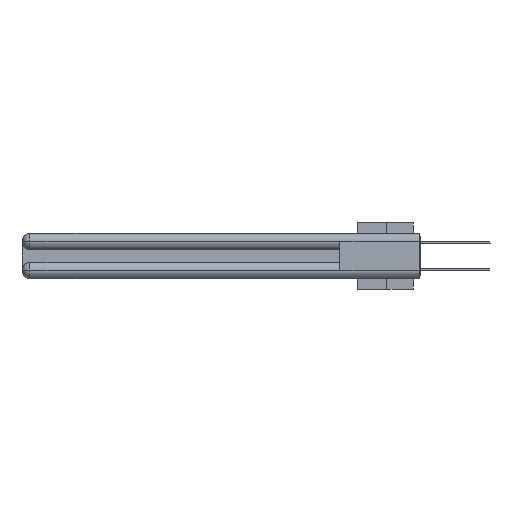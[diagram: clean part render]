
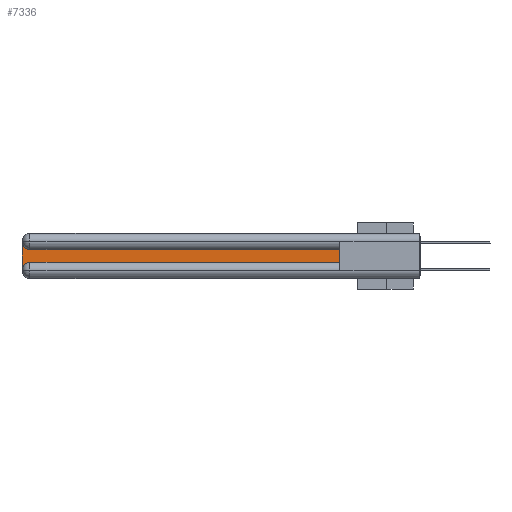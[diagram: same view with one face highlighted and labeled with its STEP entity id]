
A CAD part, left-side view. The second image highlights one B-rep face of the part: STEP entity #7336.
In plain terms, the highlighted planar face has unit normal (-1, 0, 0).
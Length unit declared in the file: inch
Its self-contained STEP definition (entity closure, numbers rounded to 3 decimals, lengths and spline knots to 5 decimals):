
#3 = DIRECTION ( 'NONE',  ( 0., 0., 1. ) ) ;
#573 = DIRECTION ( 'NONE',  ( 0., 1., 0. ) ) ;
#1075 = LINE ( 'NONE', #16398, #37782 ) ;
#2885 = DIRECTION ( 'NONE',  ( 0., 0., -1. ) ) ;
#3100 = DIRECTION ( 'NONE',  ( 1., 0., 0. ) ) ;
#4348 = LINE ( 'NONE', #16305, #14561 ) ;
#4958 = EDGE_CURVE ( 'NONE', #39099, #21110, #28471, .T. ) ;
#5521 = DIRECTION ( 'NONE',  ( 0., 0., -1. ) ) ;
#5944 = DIRECTION ( 'NONE',  ( 1., 0., 0. ) ) ;
#6225 = CARTESIAN_POINT ( 'NONE',  ( 0.075, 2.94, -0.2775 ) ) ;
#7336 = ADVANCED_FACE ( 'NONE', ( #25384 ), #31634, .F. ) ;
#8927 = VECTOR ( 'NONE', #3, 39.37008 ) ;
#10558 = CARTESIAN_POINT ( 'NONE',  ( 0.075, 0.6, -0.2175 ) ) ;
#14336 = EDGE_CURVE ( 'NONE', #37488, #26446, #1075, .T. ) ;
#14561 = VECTOR ( 'NONE', #573, 39.37008 ) ;
#15164 = VECTOR ( 'NONE', #25741, 39.37008 ) ;
#16305 = CARTESIAN_POINT ( 'NONE',  ( 0.075, 0.6, -0.1225 ) ) ;
#16398 = CARTESIAN_POINT ( 'NONE',  ( 0.075, 0.6, -0.2175 ) ) ;
#16841 = EDGE_CURVE ( 'NONE', #24533, #39099, #22353, .T. ) ;
#17554 = AXIS2_PLACEMENT_3D ( 'NONE', #6225, #3100, #20787 ) ;
#17930 = CARTESIAN_POINT ( 'NONE',  ( 0.075, 2.94, -0.0625 ) ) ;
#18009 = EDGE_CURVE ( 'NONE', #19105, #24533, #4348, .T. ) ;
#18249 = ORIENTED_EDGE ( 'NONE', *, *, #37626, .T. ) ;
#18972 = AXIS2_PLACEMENT_3D ( 'NONE', #17930, #5944, #5521 ) ;
#19105 = VERTEX_POINT ( 'NONE', #32090 ) ;
#19639 = CARTESIAN_POINT ( 'NONE',  ( 0.075, 3., -0.2775 ) ) ;
#19967 = CARTESIAN_POINT ( 'NONE',  ( 0.075, 2.94, -0.2175 ) ) ;
#20294 = AXIS2_PLACEMENT_3D ( 'NONE', #24542, #21560, #2885 ) ;
#20787 = DIRECTION ( 'NONE',  ( 0., 0., -1. ) ) ;
#20843 = EDGE_LOOP ( 'NONE', ( #36599, #25757, #38647, #18249, #28880, #35596 ) ) ;
#21110 = VERTEX_POINT ( 'NONE', #19639 ) ;
#21560 = DIRECTION ( 'NONE',  ( 1., 0., 0. ) ) ;
#22169 = CARTESIAN_POINT ( 'NONE',  ( 0.075, 2.94, -0.1225 ) ) ;
#22353 = CIRCLE ( 'NONE', #18972, 0.06 ) ;
#24533 = VERTEX_POINT ( 'NONE', #22169 ) ;
#24542 = CARTESIAN_POINT ( 'NONE',  ( 0.075, 3., -0.1225 ) ) ;
#25228 = CARTESIAN_POINT ( 'NONE',  ( 0.075, 0.6, -0.2175 ) ) ;
#25384 = FACE_OUTER_BOUND ( 'NONE', #20843, .T. ) ;
#25741 = DIRECTION ( 'NONE',  ( 0., 0., -1. ) ) ;
#25757 = ORIENTED_EDGE ( 'NONE', *, *, #16841, .T. ) ;
#26055 = LINE ( 'NONE', #25228, #8927 ) ;
#26446 = VERTEX_POINT ( 'NONE', #10558 ) ;
#28471 = LINE ( 'NONE', #41293, #15164 ) ;
#28880 = ORIENTED_EDGE ( 'NONE', *, *, #14336, .T. ) ;
#28954 = CIRCLE ( 'NONE', #17554, 0.06 ) ;
#31634 = PLANE ( 'NONE',  #20294 ) ;
#32090 = CARTESIAN_POINT ( 'NONE',  ( 0.075, 0.6, -0.1225 ) ) ;
#33765 = DIRECTION ( 'NONE',  ( 0., -1., 0. ) ) ;
#35058 = CARTESIAN_POINT ( 'NONE',  ( 0.075, 3., -0.0625 ) ) ;
#35596 = ORIENTED_EDGE ( 'NONE', *, *, #39058, .T. ) ;
#36599 = ORIENTED_EDGE ( 'NONE', *, *, #18009, .T. ) ;
#37488 = VERTEX_POINT ( 'NONE', #19967 ) ;
#37626 = EDGE_CURVE ( 'NONE', #21110, #37488, #28954, .T. ) ;
#37782 = VECTOR ( 'NONE', #33765, 39.37008 ) ;
#38647 = ORIENTED_EDGE ( 'NONE', *, *, #4958, .T. ) ;
#39058 = EDGE_CURVE ( 'NONE', #26446, #19105, #26055, .T. ) ;
#39099 = VERTEX_POINT ( 'NONE', #35058 ) ;
#41293 = CARTESIAN_POINT ( 'NONE',  ( 0.075, 3., -0.2175 ) ) ;
